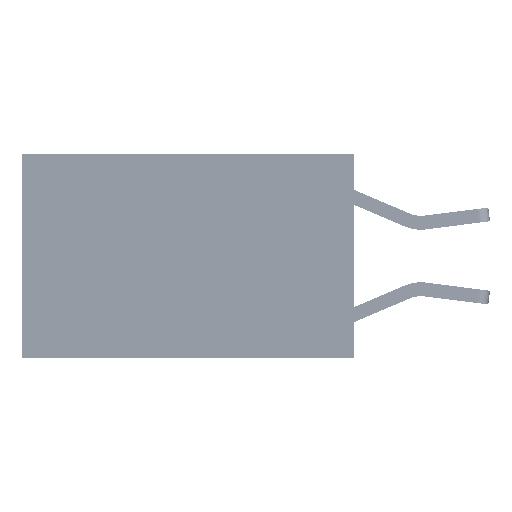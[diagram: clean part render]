
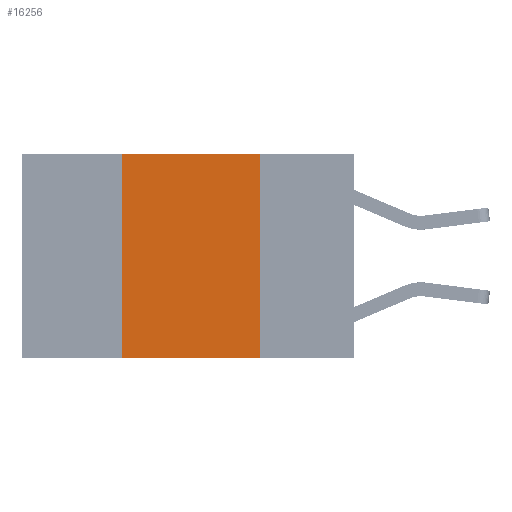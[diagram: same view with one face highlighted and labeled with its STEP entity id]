
A CAD part, left-side view. The second image highlights one B-rep face of the part: STEP entity #16256.
In plain terms, the highlighted planar face has unit normal (-1, 0, 0).
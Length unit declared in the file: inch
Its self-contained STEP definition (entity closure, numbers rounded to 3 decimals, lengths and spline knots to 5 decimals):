
#582 = VERTEX_POINT ( 'NONE', #6395 ) ;
#835 = CARTESIAN_POINT ( 'NONE',  ( 0., 0.6, 0. ) ) ;
#2144 = VERTEX_POINT ( 'NONE', #31860 ) ;
#2211 = CARTESIAN_POINT ( 'NONE',  ( 0., 0.6, 0. ) ) ;
#2234 = VERTEX_POINT ( 'NONE', #7679 ) ;
#2939 = ORIENTED_EDGE ( 'NONE', *, *, #3685, .F. ) ;
#3685 = EDGE_CURVE ( 'NONE', #2234, #582, #23143, .T. ) ;
#6395 = CARTESIAN_POINT ( 'NONE',  ( 0., 0.17, 0. ) ) ;
#7218 = DIRECTION ( 'NONE',  ( 0., 0., -1. ) ) ;
#7351 = VERTEX_POINT ( 'NONE', #16533 ) ;
#7479 = DIRECTION ( 'NONE',  ( 0., 0., 1. ) ) ;
#7679 = CARTESIAN_POINT ( 'NONE',  ( 0., 0.42, 0. ) ) ;
#10345 = ORIENTED_EDGE ( 'NONE', *, *, #31407, .F. ) ;
#10875 = DIRECTION ( 'NONE',  ( 0., -1., 0. ) ) ;
#11327 = EDGE_LOOP ( 'NONE', ( #26934, #2939, #10345, #30786 ) ) ;
#12221 = AXIS2_PLACEMENT_3D ( 'NONE', #2211, #22027, #7218 ) ;
#12224 = EDGE_CURVE ( 'NONE', #2144, #7351, #21858, .T. ) ;
#12256 = CARTESIAN_POINT ( 'NONE',  ( 0., 0.6, -0.37 ) ) ;
#12358 = FACE_OUTER_BOUND ( 'NONE', #11327, .T. ) ;
#12525 = VECTOR ( 'NONE', #7479, 39.37008 ) ;
#13834 = CARTESIAN_POINT ( 'NONE',  ( 0., 0.17, 0. ) ) ;
#16256 = ADVANCED_FACE ( 'NONE', ( #12358 ), #19548, .F. ) ;
#16316 = DIRECTION ( 'NONE',  ( 0., 0., -1. ) ) ;
#16533 = CARTESIAN_POINT ( 'NONE',  ( 0., 0.17, -0.37 ) ) ;
#16612 = VECTOR ( 'NONE', #10875, 39.37008 ) ;
#19548 = PLANE ( 'NONE',  #12221 ) ;
#19686 = DIRECTION ( 'NONE',  ( 0., -1., 0. ) ) ;
#19862 = EDGE_CURVE ( 'NONE', #582, #7351, #24291, .T. ) ;
#21858 = LINE ( 'NONE', #12256, #27651 ) ;
#22027 = DIRECTION ( 'NONE',  ( 1., 0., 0. ) ) ;
#22281 = CARTESIAN_POINT ( 'NONE',  ( 0., 0.42, 0. ) ) ;
#23143 = LINE ( 'NONE', #835, #16612 ) ;
#24291 = LINE ( 'NONE', #13834, #28512 ) ;
#26934 = ORIENTED_EDGE ( 'NONE', *, *, #19862, .F. ) ;
#27651 = VECTOR ( 'NONE', #19686, 39.37008 ) ;
#28512 = VECTOR ( 'NONE', #16316, 39.37008 ) ;
#30786 = ORIENTED_EDGE ( 'NONE', *, *, #12224, .T. ) ;
#31383 = LINE ( 'NONE', #22281, #12525 ) ;
#31407 = EDGE_CURVE ( 'NONE', #2144, #2234, #31383, .T. ) ;
#31860 = CARTESIAN_POINT ( 'NONE',  ( 0., 0.42, -0.37 ) ) ;
